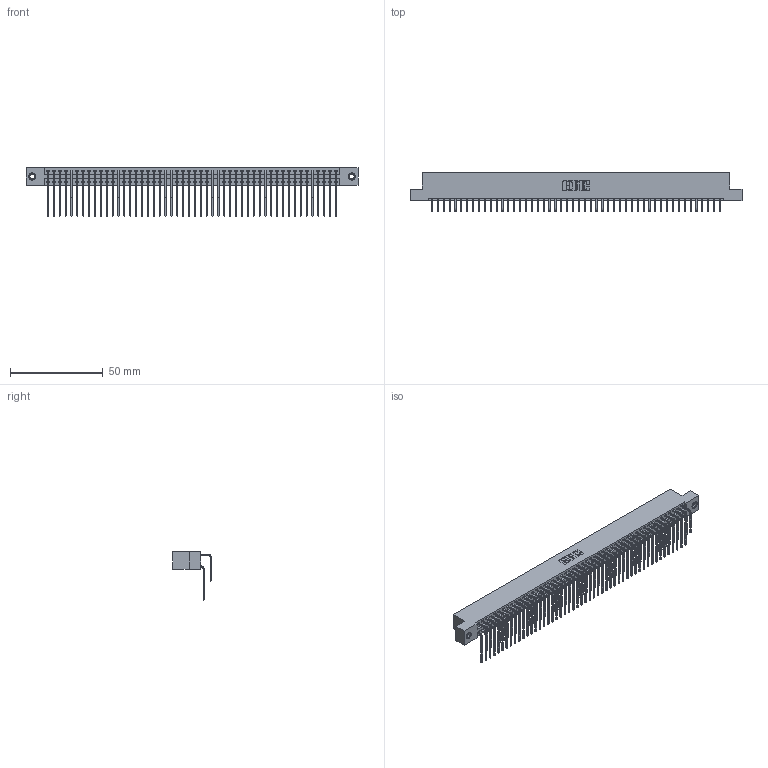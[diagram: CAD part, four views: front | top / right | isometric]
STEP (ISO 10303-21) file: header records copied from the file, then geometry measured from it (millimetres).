
FILE_DESCRIPTION (( 'STEP AP203' ), '1' );
FILE_NAME ('396-100-559-207.STEP', '2019-11-03T16:09:41', ( '' ), ( '' ), 'SwSTEP 2.0', 'SolidWorks 2016', '' );
FILE_SCHEMA (( 'CONFIG_CONTROL_DESIGN' ));
Length unit declared in the file: inch
Products named in the file (5): 345-292-001_558 559 Tail - 1; 396-100-559-207; 345-250-001_345-250-005-103; 346 Part_Flush Mounting Lugs - 0.156 Dia-TI; 345-292-001_559 Tail - 2
Assembly tree (103 placements, depth 2):
  396-100-559-207
    346 Part_Flush Mounting Lugs - 0.156 Dia-TI
    345-292-001_558 559 Tail - 1  x50
    345-292-001_559 Tail - 2  x50
    345-250-001_345-250-005-103  x2
Bounding box: 179.32 x 20.89 x 26.16 mm (x, y, z)
Volume: 18111.8 mm3; surface area: 27822.9 mm2
Topology: 103 solids, 103 shells, 5582 faces, 16565 edges, 10902 vertices
Faces by surface type: plane 3808, cylinder 1758, cone 12, torus 4
Entity records: 34524 total; most frequent: CARTESIAN_POINT 5714, ORIENTED_EDGE 5590, DIRECTION 5085, EDGE_CURVE 2795, LINE 2403, VECTOR 2403, VERTEX_POINT 1856, AXIS2_PLACEMENT_3D 1341
